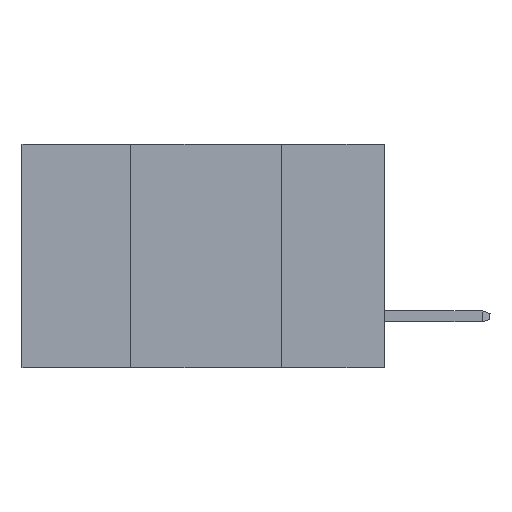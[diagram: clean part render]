
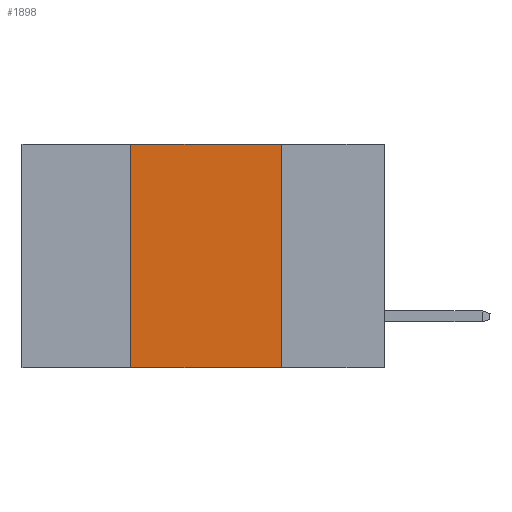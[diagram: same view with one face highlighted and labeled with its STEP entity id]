
A CAD part, left-side view. The second image highlights one B-rep face of the part: STEP entity #1898.
In plain terms, the highlighted planar face has unit normal (-1, 0, 0).
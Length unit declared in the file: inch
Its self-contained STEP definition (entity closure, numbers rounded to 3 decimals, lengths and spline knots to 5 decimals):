
#1843 = LINE ( 'NONE', #3652, #16346 ) ;
#1896 = ORIENTED_EDGE ( 'NONE', *, *, #4774, .F. ) ;
#1898 = ADVANCED_FACE ( 'NONE', ( #7081 ), #3544, .F. ) ;
#2625 = LINE ( 'NONE', #18165, #14033 ) ;
#3544 = PLANE ( 'NONE',  #5413 ) ;
#3611 = DIRECTION ( 'NONE',  ( 1., 0., 0. ) ) ;
#3652 = CARTESIAN_POINT ( 'NONE',  ( 0., 0.42, 0. ) ) ;
#4560 = CARTESIAN_POINT ( 'NONE',  ( 0., 0.17, -0.37 ) ) ;
#4774 = EDGE_CURVE ( 'NONE', #9298, #16332, #1843, .T. ) ;
#4973 = DIRECTION ( 'NONE',  ( 0., 0., 1. ) ) ;
#5086 = VERTEX_POINT ( 'NONE', #7109 ) ;
#5413 = AXIS2_PLACEMENT_3D ( 'NONE', #6615, #3611, #17885 ) ;
#5463 = LINE ( 'NONE', #15728, #14842 ) ;
#5496 = CARTESIAN_POINT ( 'NONE',  ( 0., 0.42, 0. ) ) ;
#5575 = EDGE_LOOP ( 'NONE', ( #8771, #14547, #1896, #7107 ) ) ;
#5907 = LINE ( 'NONE', #17695, #6117 ) ;
#6117 = VECTOR ( 'NONE', #17633, 39.37008 ) ;
#6615 = CARTESIAN_POINT ( 'NONE',  ( 0., 0.6, 0. ) ) ;
#6653 = DIRECTION ( 'NONE',  ( 0., -1., 0. ) ) ;
#7081 = FACE_OUTER_BOUND ( 'NONE', #5575, .T. ) ;
#7107 = ORIENTED_EDGE ( 'NONE', *, *, #15128, .T. ) ;
#7109 = CARTESIAN_POINT ( 'NONE',  ( 0., 0.17, 0. ) ) ;
#8771 = ORIENTED_EDGE ( 'NONE', *, *, #10630, .F. ) ;
#9298 = VERTEX_POINT ( 'NONE', #14110 ) ;
#10630 = EDGE_CURVE ( 'NONE', #5086, #12808, #5463, .T. ) ;
#12808 = VERTEX_POINT ( 'NONE', #4560 ) ;
#14033 = VECTOR ( 'NONE', #6653, 39.37008 ) ;
#14110 = CARTESIAN_POINT ( 'NONE',  ( 0., 0.42, -0.37 ) ) ;
#14547 = ORIENTED_EDGE ( 'NONE', *, *, #17980, .F. ) ;
#14842 = VECTOR ( 'NONE', #16971, 39.37008 ) ;
#15128 = EDGE_CURVE ( 'NONE', #9298, #12808, #2625, .T. ) ;
#15728 = CARTESIAN_POINT ( 'NONE',  ( 0., 0.17, 0. ) ) ;
#16332 = VERTEX_POINT ( 'NONE', #5496 ) ;
#16346 = VECTOR ( 'NONE', #4973, 39.37008 ) ;
#16971 = DIRECTION ( 'NONE',  ( 0., 0., -1. ) ) ;
#17633 = DIRECTION ( 'NONE',  ( 0., -1., 0. ) ) ;
#17695 = CARTESIAN_POINT ( 'NONE',  ( 0., 0.6, 0. ) ) ;
#17885 = DIRECTION ( 'NONE',  ( 0., 0., -1. ) ) ;
#17980 = EDGE_CURVE ( 'NONE', #16332, #5086, #5907, .T. ) ;
#18165 = CARTESIAN_POINT ( 'NONE',  ( 0., 0.6, -0.37 ) ) ;
